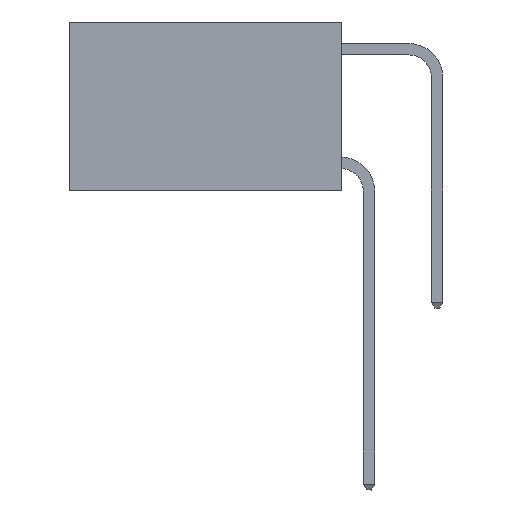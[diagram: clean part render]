
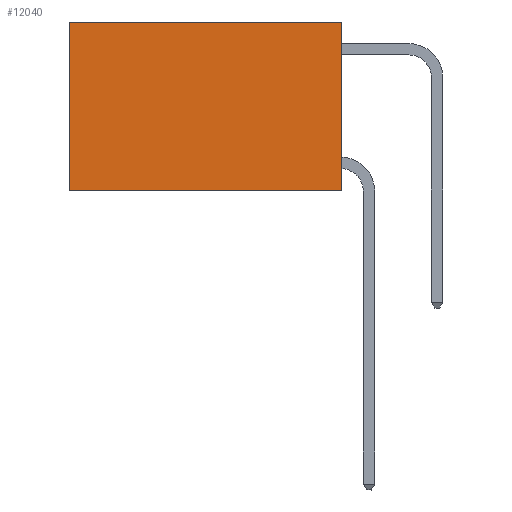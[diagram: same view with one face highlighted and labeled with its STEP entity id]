
A CAD part, left-side view. The second image highlights one B-rep face of the part: STEP entity #12040.
In plain terms, the highlighted planar face has unit normal (-1, 0, 0).
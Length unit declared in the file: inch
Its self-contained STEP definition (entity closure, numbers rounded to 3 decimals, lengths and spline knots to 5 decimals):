
#102 = LINE ( 'NONE', #7924, #12183 ) ;
#142 = VERTEX_POINT ( 'NONE', #17962 ) ;
#343 = DIRECTION ( 'NONE',  ( 0., 0., -1. ) ) ;
#724 = CARTESIAN_POINT ( 'NONE',  ( 0.2625, 0.6, 0. ) ) ;
#1126 = FACE_OUTER_BOUND ( 'NONE', #10246, .T. ) ;
#2979 = CARTESIAN_POINT ( 'NONE',  ( 0.2625, 0., -0.37 ) ) ;
#3713 = EDGE_CURVE ( 'NONE', #5860, #17478, #102, .T. ) ;
#4366 = CARTESIAN_POINT ( 'NONE',  ( 0.2625, 0., 0. ) ) ;
#5482 = DIRECTION ( 'NONE',  ( 0., 1., 0. ) ) ;
#5498 = DIRECTION ( 'NONE',  ( 0., 0., -1. ) ) ;
#5860 = VERTEX_POINT ( 'NONE', #724 ) ;
#6724 = AXIS2_PLACEMENT_3D ( 'NONE', #17077, #14769, #343 ) ;
#7924 = CARTESIAN_POINT ( 'NONE',  ( 0.2625, 0.6, 0. ) ) ;
#8390 = VECTOR ( 'NONE', #5482, 39.37008 ) ;
#9971 = CARTESIAN_POINT ( 'NONE',  ( 0.2625, 0.6, -0.37 ) ) ;
#10246 = EDGE_LOOP ( 'NONE', ( #14249, #12096, #26365, #17108 ) ) ;
#12040 = ADVANCED_FACE ( 'NONE', ( #1126 ), #29034, .F. ) ;
#12096 = ORIENTED_EDGE ( 'NONE', *, *, #17038, .F. ) ;
#12183 = VECTOR ( 'NONE', #5498, 39.37008 ) ;
#14249 = ORIENTED_EDGE ( 'NONE', *, *, #3713, .T. ) ;
#14769 = DIRECTION ( 'NONE',  ( 1., 0., 0. ) ) ;
#14806 = LINE ( 'NONE', #2979, #8390 ) ;
#16474 = DIRECTION ( 'NONE',  ( 0., 1., 0. ) ) ;
#17038 = EDGE_CURVE ( 'NONE', #142, #17478, #14806, .T. ) ;
#17077 = CARTESIAN_POINT ( 'NONE',  ( 0.2625, 0., 0. ) ) ;
#17108 = ORIENTED_EDGE ( 'NONE', *, *, #26532, .T. ) ;
#17478 = VERTEX_POINT ( 'NONE', #9971 ) ;
#17962 = CARTESIAN_POINT ( 'NONE',  ( 0.2625, 0., -0.37 ) ) ;
#19576 = VECTOR ( 'NONE', #28321, 39.37008 ) ;
#22137 = EDGE_CURVE ( 'NONE', #27027, #142, #25905, .T. ) ;
#25905 = LINE ( 'NONE', #4366, #19576 ) ;
#26365 = ORIENTED_EDGE ( 'NONE', *, *, #22137, .F. ) ;
#26532 = EDGE_CURVE ( 'NONE', #27027, #5860, #27969, .T. ) ;
#26732 = CARTESIAN_POINT ( 'NONE',  ( 0.2625, 0., 0. ) ) ;
#27027 = VERTEX_POINT ( 'NONE', #26732 ) ;
#27969 = LINE ( 'NONE', #28346, #28718 ) ;
#28321 = DIRECTION ( 'NONE',  ( 0., 0., -1. ) ) ;
#28346 = CARTESIAN_POINT ( 'NONE',  ( 0.2625, 0., 0. ) ) ;
#28718 = VECTOR ( 'NONE', #16474, 39.37008 ) ;
#29034 = PLANE ( 'NONE',  #6724 ) ;
